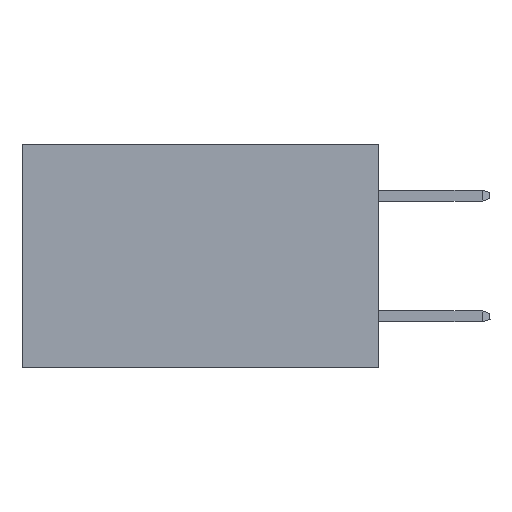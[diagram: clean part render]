
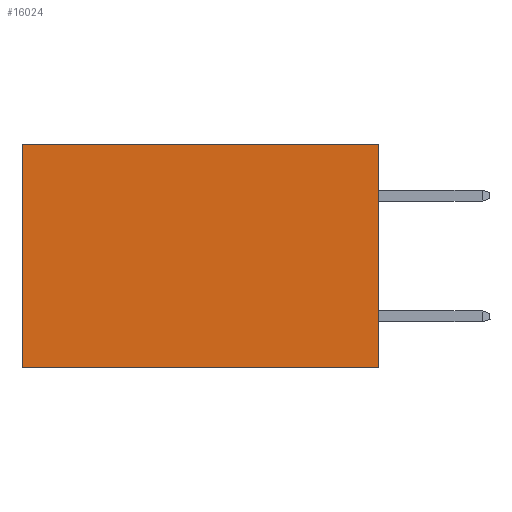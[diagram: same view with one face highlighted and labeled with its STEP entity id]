
A CAD part, left-side view. The second image highlights one B-rep face of the part: STEP entity #16024.
In plain terms, the highlighted planar face has unit normal (-1, 0, 0).
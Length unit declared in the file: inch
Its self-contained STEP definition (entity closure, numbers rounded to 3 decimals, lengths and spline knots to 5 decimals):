
#1595 = CARTESIAN_POINT ( 'NONE',  ( 0.277, 0.59, -0.37 ) ) ;
#1661 = VERTEX_POINT ( 'NONE', #16301 ) ;
#1769 = ORIENTED_EDGE ( 'NONE', *, *, #11269, .F. ) ;
#2857 = ORIENTED_EDGE ( 'NONE', *, *, #13506, .T. ) ;
#3287 = CARTESIAN_POINT ( 'NONE',  ( 0.277, 0.59, -0.37 ) ) ;
#3579 = FACE_OUTER_BOUND ( 'NONE', #13672, .T. ) ;
#3782 = CARTESIAN_POINT ( 'NONE',  ( 0.277, 0., 0. ) ) ;
#5006 = DIRECTION ( 'NONE',  ( 0., 0., -1. ) ) ;
#5050 = CARTESIAN_POINT ( 'NONE',  ( 0.277, 0., -0.37 ) ) ;
#5501 = DIRECTION ( 'NONE',  ( 0., 1., 0. ) ) ;
#5507 = CARTESIAN_POINT ( 'NONE',  ( 0.277, 0., -0.37 ) ) ;
#5716 = ORIENTED_EDGE ( 'NONE', *, *, #7885, .F. ) ;
#6106 = CARTESIAN_POINT ( 'NONE',  ( 0.277, 0., -0.37 ) ) ;
#6751 = DIRECTION ( 'NONE',  ( 0., 1., 0. ) ) ;
#6773 = CARTESIAN_POINT ( 'NONE',  ( 0.277, 0., -0.37 ) ) ;
#7109 = PLANE ( 'NONE',  #16023 ) ;
#7197 = DIRECTION ( 'NONE',  ( 0., 0., -1. ) ) ;
#7582 = VECTOR ( 'NONE', #5006, 39.37008 ) ;
#7885 = EDGE_CURVE ( 'NONE', #17060, #9278, #9057, .T. ) ;
#8125 = LINE ( 'NONE', #3287, #7582 ) ;
#9057 = LINE ( 'NONE', #5050, #17338 ) ;
#9278 = VERTEX_POINT ( 'NONE', #1595 ) ;
#9345 = VERTEX_POINT ( 'NONE', #16777 ) ;
#11269 = EDGE_CURVE ( 'NONE', #9345, #17060, #21329, .T. ) ;
#11344 = VECTOR ( 'NONE', #5501, 39.37008 ) ;
#11865 = DIRECTION ( 'NONE',  ( 0., 0., -1. ) ) ;
#11964 = ORIENTED_EDGE ( 'NONE', *, *, #21444, .T. ) ;
#13506 = EDGE_CURVE ( 'NONE', #9345, #1661, #20133, .T. ) ;
#13672 = EDGE_LOOP ( 'NONE', ( #11964, #5716, #1769, #2857 ) ) ;
#16024 = ADVANCED_FACE ( 'NONE', ( #3579 ), #7109, .F. ) ;
#16023 = AXIS2_PLACEMENT_3D ( 'NONE', #5507, #17140, #7197 ) ;
#16301 = CARTESIAN_POINT ( 'NONE',  ( 0.277, 0.59, 0. ) ) ;
#16777 = CARTESIAN_POINT ( 'NONE',  ( 0.277, 0., 0. ) ) ;
#16922 = VECTOR ( 'NONE', #11865, 39.37008 ) ;
#17060 = VERTEX_POINT ( 'NONE', #6106 ) ;
#17140 = DIRECTION ( 'NONE',  ( 1., 0., 0. ) ) ;
#17338 = VECTOR ( 'NONE', #6751, 39.37008 ) ;
#20133 = LINE ( 'NONE', #3782, #11344 ) ;
#21329 = LINE ( 'NONE', #6773, #16922 ) ;
#21444 = EDGE_CURVE ( 'NONE', #1661, #9278, #8125, .T. ) ;
